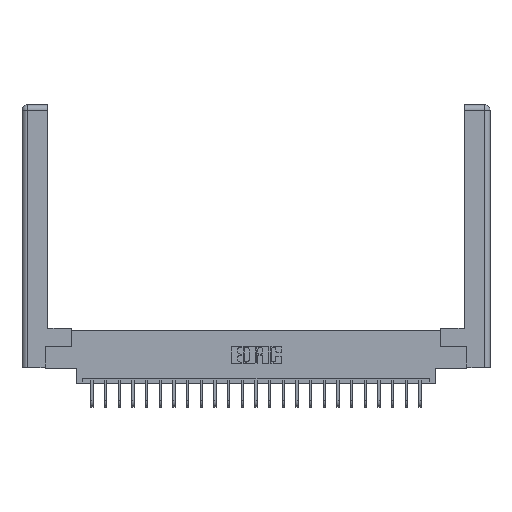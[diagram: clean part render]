
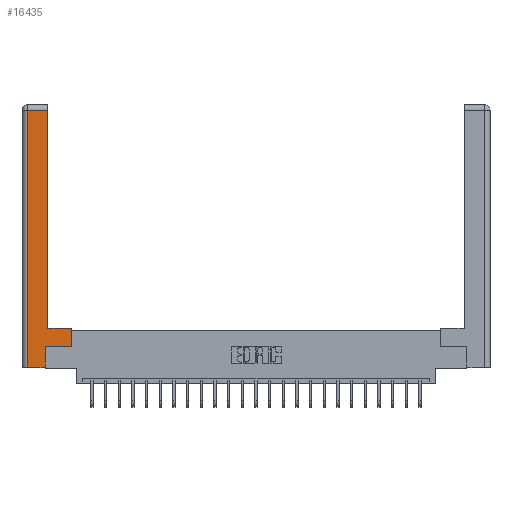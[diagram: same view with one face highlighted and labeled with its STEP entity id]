
A CAD part, top view. The second image highlights one B-rep face of the part: STEP entity #16435.
In plain terms, the highlighted planar face has unit normal (0, 0, 1).
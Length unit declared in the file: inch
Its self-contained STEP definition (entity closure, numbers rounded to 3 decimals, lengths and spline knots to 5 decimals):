
#379 = DIRECTION ( 'NONE',  ( 0., 1., 0. ) ) ;
#1156 = CARTESIAN_POINT ( 'NONE',  ( 0.295, 3., 0. ) ) ;
#1677 = EDGE_CURVE ( 'NONE', #15850, #1752, #7463, .T. ) ;
#1752 = VERTEX_POINT ( 'NONE', #14103 ) ;
#2668 = VECTOR ( 'NONE', #20446, 39.37008 ) ;
#4595 = DIRECTION ( 'NONE',  ( 1., 0., 0. ) ) ;
#4842 = VECTOR ( 'NONE', #4595, 39.37008 ) ;
#5799 = EDGE_CURVE ( 'NONE', #9822, #15850, #22404, .T. ) ;
#5972 = CARTESIAN_POINT ( 'NONE',  ( 0.295, 0.45, 0. ) ) ;
#6102 = ORIENTED_EDGE ( 'NONE', *, *, #19654, .T. ) ;
#6136 = VECTOR ( 'NONE', #379, 39.37008 ) ;
#6202 = VECTOR ( 'NONE', #15023, 39.37008 ) ;
#6451 = CARTESIAN_POINT ( 'NONE',  ( 0.0615, 2.94, 0. ) ) ;
#6618 = VECTOR ( 'NONE', #17292, 39.37008 ) ;
#6693 = CARTESIAN_POINT ( 'NONE',  ( 0., 0., 0. ) ) ;
#6706 = LINE ( 'NONE', #20718, #6136 ) ;
#6797 = CARTESIAN_POINT ( 'NONE',  ( 0.0615, 0., 0. ) ) ;
#6923 = PLANE ( 'NONE',  #16377 ) ;
#7087 = EDGE_CURVE ( 'NONE', #10302, #16560, #9812, .T. ) ;
#7463 = LINE ( 'NONE', #15470, #6618 ) ;
#7507 = DIRECTION ( 'NONE',  ( 0., 1., 0. ) ) ;
#8965 = VECTOR ( 'NONE', #13745, 39.37008 ) ;
#9318 = ORIENTED_EDGE ( 'NONE', *, *, #1677, .T. ) ;
#9380 = VECTOR ( 'NONE', #7507, 39.37008 ) ;
#9812 = LINE ( 'NONE', #5972, #2668 ) ;
#9822 = VERTEX_POINT ( 'NONE', #11604 ) ;
#9835 = ORIENTED_EDGE ( 'NONE', *, *, #7087, .T. ) ;
#10302 = VERTEX_POINT ( 'NONE', #16464 ) ;
#10536 = DIRECTION ( 'NONE',  ( 0., 0., -1. ) ) ;
#11378 = CARTESIAN_POINT ( 'NONE',  ( 0.265, 0.245, 0. ) ) ;
#11604 = CARTESIAN_POINT ( 'NONE',  ( 0.265, 0., 0. ) ) ;
#11871 = CARTESIAN_POINT ( 'NONE',  ( 0.295, 2.94, 0. ) ) ;
#12501 = LINE ( 'NONE', #13364, #6202 ) ;
#12768 = VERTEX_POINT ( 'NONE', #6797 ) ;
#13364 = CARTESIAN_POINT ( 'NONE',  ( 0.0615, 0., 0. ) ) ;
#13432 = EDGE_LOOP ( 'NONE', ( #18584, #18506, #6102, #21071, #19790, #9318, #23264, #9835 ) ) ;
#13745 = DIRECTION ( 'NONE',  ( -1., 0., 0. ) ) ;
#13834 = LINE ( 'NONE', #6451, #8965 ) ;
#14103 = CARTESIAN_POINT ( 'NONE',  ( 0.565, 0.245, 0. ) ) ;
#14283 = VERTEX_POINT ( 'NONE', #16162 ) ;
#15023 = DIRECTION ( 'NONE',  ( 0., -1., 0. ) ) ;
#15470 = CARTESIAN_POINT ( 'NONE',  ( 0.565, 0.245, 0. ) ) ;
#15478 = EDGE_CURVE ( 'NONE', #12768, #9822, #23109, .T. ) ;
#15533 = CARTESIAN_POINT ( 'NONE',  ( 0.265, 0., 0. ) ) ;
#15850 = VERTEX_POINT ( 'NONE', #11378 ) ;
#16114 = EDGE_CURVE ( 'NONE', #16560, #17351, #22798, .T. ) ;
#16162 = CARTESIAN_POINT ( 'NONE',  ( 0.0615, 2.94, 0. ) ) ;
#16377 = AXIS2_PLACEMENT_3D ( 'NONE', #6693, #10536, #23300 ) ;
#16435 = ADVANCED_FACE ( 'NONE', ( #18785 ), #6923, .F. ) ;
#16464 = CARTESIAN_POINT ( 'NONE',  ( 0.565, 0.45, 0. ) ) ;
#16560 = VERTEX_POINT ( 'NONE', #18504 ) ;
#16996 = CARTESIAN_POINT ( 'NONE',  ( 0.265, 0.245, 0. ) ) ;
#17292 = DIRECTION ( 'NONE',  ( 1., 0., 0. ) ) ;
#17351 = VERTEX_POINT ( 'NONE', #11871 ) ;
#18504 = CARTESIAN_POINT ( 'NONE',  ( 0.295, 0.45, 0. ) ) ;
#18506 = ORIENTED_EDGE ( 'NONE', *, *, #21660, .T. ) ;
#18584 = ORIENTED_EDGE ( 'NONE', *, *, #16114, .T. ) ;
#18785 = FACE_OUTER_BOUND ( 'NONE', #13432, .T. ) ;
#19654 = EDGE_CURVE ( 'NONE', #14283, #12768, #12501, .T. ) ;
#19790 = ORIENTED_EDGE ( 'NONE', *, *, #5799, .T. ) ;
#20446 = DIRECTION ( 'NONE',  ( -1., 0., 0. ) ) ;
#20659 = DIRECTION ( 'NONE',  ( 0., 1., 0. ) ) ;
#20701 = VECTOR ( 'NONE', #20659, 39.37008 ) ;
#20718 = CARTESIAN_POINT ( 'NONE',  ( 0.565, 0.45, 0. ) ) ;
#20881 = EDGE_CURVE ( 'NONE', #1752, #10302, #6706, .T. ) ;
#21071 = ORIENTED_EDGE ( 'NONE', *, *, #15478, .T. ) ;
#21660 = EDGE_CURVE ( 'NONE', #17351, #14283, #13834, .T. ) ;
#22404 = LINE ( 'NONE', #16996, #20701 ) ;
#22798 = LINE ( 'NONE', #1156, #9380 ) ;
#23109 = LINE ( 'NONE', #15533, #4842 ) ;
#23264 = ORIENTED_EDGE ( 'NONE', *, *, #20881, .T. ) ;
#23300 = DIRECTION ( 'NONE',  ( -1., 0., 0. ) ) ;
